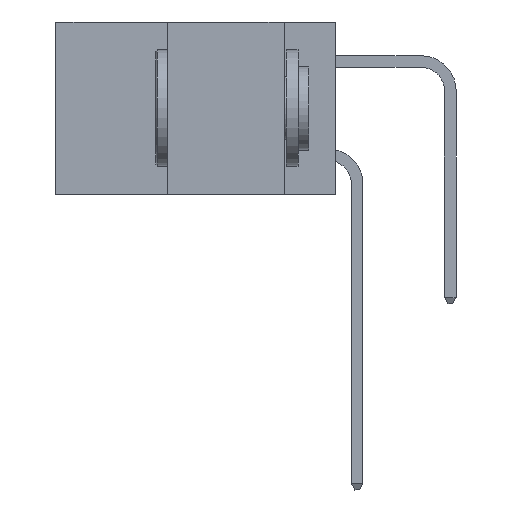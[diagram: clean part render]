
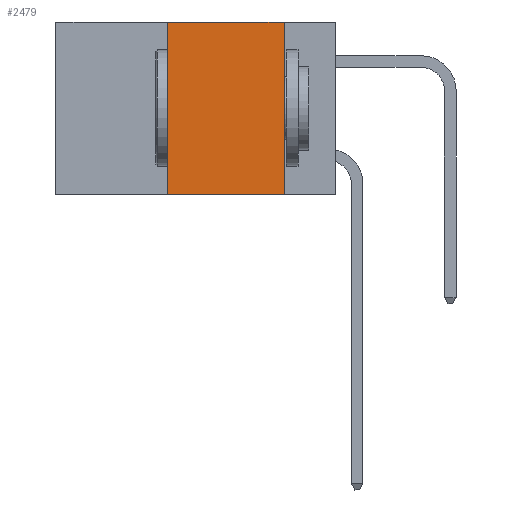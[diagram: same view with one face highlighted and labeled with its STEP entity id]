
A CAD part, left-side view. The second image highlights one B-rep face of the part: STEP entity #2479.
In plain terms, the highlighted planar face has unit normal (-1, 0, 0).
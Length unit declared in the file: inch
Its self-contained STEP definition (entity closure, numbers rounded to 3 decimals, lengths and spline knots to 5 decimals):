
#1227 = CARTESIAN_POINT ( 'NONE',  ( 0., 0.6, 0. ) ) ;
#2001 = EDGE_LOOP ( 'NONE', ( #2769, #5361, #19213, #6039 ) ) ;
#2479 = ADVANCED_FACE ( 'NONE', ( #11938 ), #9135, .F. ) ;
#2769 = ORIENTED_EDGE ( 'NONE', *, *, #3842, .F. ) ;
#3842 = EDGE_CURVE ( 'NONE', #7788, #13635, #10157, .T. ) ;
#4463 = DIRECTION ( 'NONE',  ( 0., 0., -1. ) ) ;
#5344 = VECTOR ( 'NONE', #20387, 39.37008 ) ;
#5361 = ORIENTED_EDGE ( 'NONE', *, *, #6221, .F. ) ;
#5506 = AXIS2_PLACEMENT_3D ( 'NONE', #1227, #10995, #4463 ) ;
#6039 = ORIENTED_EDGE ( 'NONE', *, *, #9092, .T. ) ;
#6221 = EDGE_CURVE ( 'NONE', #15360, #7788, #20299, .T. ) ;
#7664 = VECTOR ( 'NONE', #9750, 39.37008 ) ;
#7694 = CARTESIAN_POINT ( 'NONE',  ( 0., 0.36, 0. ) ) ;
#7788 = VERTEX_POINT ( 'NONE', #19610 ) ;
#9092 = EDGE_CURVE ( 'NONE', #11905, #13635, #14567, .T. ) ;
#9135 = PLANE ( 'NONE',  #5506 ) ;
#9750 = DIRECTION ( 'NONE',  ( 0., 0., -1. ) ) ;
#10157 = LINE ( 'NONE', #11217, #7664 ) ;
#10369 = VECTOR ( 'NONE', #11099, 39.37008 ) ;
#10995 = DIRECTION ( 'NONE',  ( 1., 0., 0. ) ) ;
#11099 = DIRECTION ( 'NONE',  ( 0., -1., 0. ) ) ;
#11217 = CARTESIAN_POINT ( 'NONE',  ( 0., 0.11, 0. ) ) ;
#11462 = VECTOR ( 'NONE', #14570, 39.37008 ) ;
#11905 = VERTEX_POINT ( 'NONE', #15660 ) ;
#11938 = FACE_OUTER_BOUND ( 'NONE', #2001, .T. ) ;
#13635 = VERTEX_POINT ( 'NONE', #14679 ) ;
#14567 = LINE ( 'NONE', #20294, #10369 ) ;
#14570 = DIRECTION ( 'NONE',  ( 0., -1., 0. ) ) ;
#14679 = CARTESIAN_POINT ( 'NONE',  ( 0., 0.11, -0.37 ) ) ;
#14861 = CARTESIAN_POINT ( 'NONE',  ( 0., 0.6, 0. ) ) ;
#15018 = LINE ( 'NONE', #15666, #5344 ) ;
#15360 = VERTEX_POINT ( 'NONE', #7694 ) ;
#15660 = CARTESIAN_POINT ( 'NONE',  ( 0., 0.36, -0.37 ) ) ;
#15666 = CARTESIAN_POINT ( 'NONE',  ( 0., 0.36, 0. ) ) ;
#19213 = ORIENTED_EDGE ( 'NONE', *, *, #19387, .F. ) ;
#19387 = EDGE_CURVE ( 'NONE', #11905, #15360, #15018, .T. ) ;
#19610 = CARTESIAN_POINT ( 'NONE',  ( 0., 0.11, 0. ) ) ;
#20294 = CARTESIAN_POINT ( 'NONE',  ( 0., 0.6, -0.37 ) ) ;
#20299 = LINE ( 'NONE', #14861, #11462 ) ;
#20387 = DIRECTION ( 'NONE',  ( 0., 0., 1. ) ) ;
